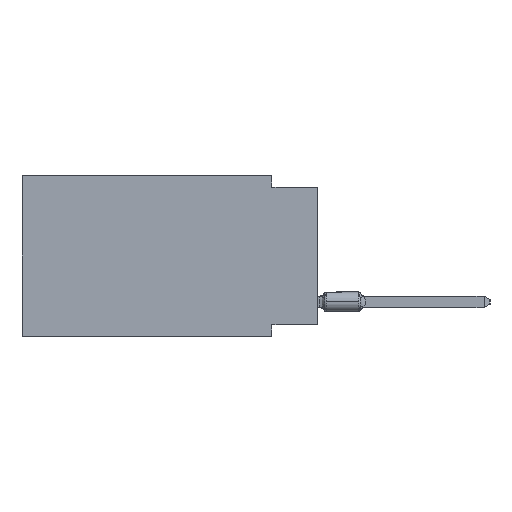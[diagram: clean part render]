
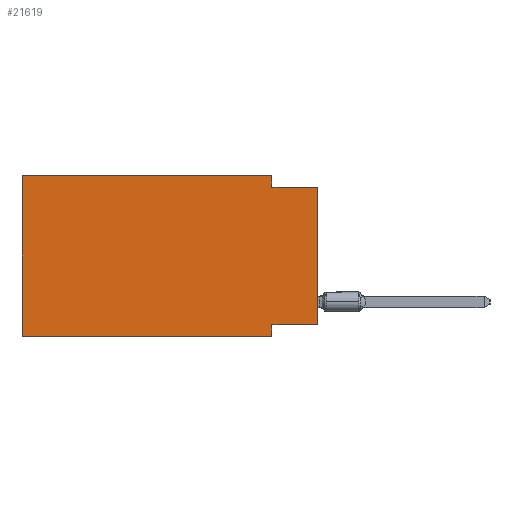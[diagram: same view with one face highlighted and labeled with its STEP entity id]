
A CAD part, left-side view. The second image highlights one B-rep face of the part: STEP entity #21619.
In plain terms, the highlighted planar face has unit normal (-1, 0, 0).
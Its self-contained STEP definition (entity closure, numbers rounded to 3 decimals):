
#1135 = VERTEX_POINT ( 'NONE', #19517 ) ;
#1807 = EDGE_CURVE ( 'NONE', #23763, #14638, #7992, .T. ) ;
#1973 = CARTESIAN_POINT ( 'NONE',  ( 0., 2.54, 0. ) ) ;
#2232 = FACE_OUTER_BOUND ( 'NONE', #28130, .T. ) ;
#3618 = DIRECTION ( 'NONE',  ( 0., 0., 1. ) ) ;
#3708 = DIRECTION ( 'NONE',  ( 0., 1., 0. ) ) ;
#3737 = VECTOR ( 'NONE', #17400, 1000. ) ;
#3788 = EDGE_CURVE ( 'NONE', #20009, #9669, #29826, .T. ) ;
#3922 = ORIENTED_EDGE ( 'NONE', *, *, #27219, .T. ) ;
#4349 = VERTEX_POINT ( 'NONE', #7233 ) ;
#4530 = ORIENTED_EDGE ( 'NONE', *, *, #3788, .T. ) ;
#4580 = VECTOR ( 'NONE', #27569, 1000. ) ;
#4931 = LINE ( 'NONE', #18668, #24850 ) ;
#5851 = VECTOR ( 'NONE', #3708, 1000. ) ;
#5910 = EDGE_CURVE ( 'NONE', #20009, #1135, #22518, .T. ) ;
#6583 = LINE ( 'NONE', #15995, #4580 ) ;
#7233 = CARTESIAN_POINT ( 'NONE',  ( 0., 2.54, -0.635 ) ) ;
#7331 = CARTESIAN_POINT ( 'NONE',  ( 0., 0., -8.255 ) ) ;
#7437 = ORIENTED_EDGE ( 'NONE', *, *, #1807, .F. ) ;
#7470 = ORIENTED_EDGE ( 'NONE', *, *, #5910, .F. ) ;
#7666 = CARTESIAN_POINT ( 'NONE',  ( 0., 16.383, 0. ) ) ;
#7992 = LINE ( 'NONE', #21720, #3737 ) ;
#8049 = ORIENTED_EDGE ( 'NONE', *, *, #16594, .F. ) ;
#8722 = LINE ( 'NONE', #25518, #11595 ) ;
#9015 = EDGE_CURVE ( 'NONE', #22147, #23763, #10734, .T. ) ;
#9669 = VERTEX_POINT ( 'NONE', #19572 ) ;
#10734 = LINE ( 'NONE', #7666, #14627 ) ;
#10968 = ORIENTED_EDGE ( 'NONE', *, *, #9015, .F. ) ;
#11595 = VECTOR ( 'NONE', #25662, 1000. ) ;
#11788 = DIRECTION ( 'NONE',  ( 1., 0., 0. ) ) ;
#12825 = EDGE_CURVE ( 'NONE', #4349, #9669, #13723, .T. ) ;
#13723 = LINE ( 'NONE', #23113, #22487 ) ;
#13924 = DIRECTION ( 'NONE',  ( 0., 0., -1. ) ) ;
#14014 = VERTEX_POINT ( 'NONE', #28874 ) ;
#14190 = DIRECTION ( 'NONE',  ( 0., -1., 0. ) ) ;
#14255 = ORIENTED_EDGE ( 'NONE', *, *, #12825, .F. ) ;
#14627 = VECTOR ( 'NONE', #17071, 1000. ) ;
#14638 = VERTEX_POINT ( 'NONE', #1973 ) ;
#15995 = CARTESIAN_POINT ( 'NONE',  ( 0., 2.54, -8.89 ) ) ;
#16594 = EDGE_CURVE ( 'NONE', #14638, #4349, #4931, .T. ) ;
#17071 = DIRECTION ( 'NONE',  ( 0., 0., 1. ) ) ;
#17400 = DIRECTION ( 'NONE',  ( 0., -1., 0. ) ) ;
#18668 = CARTESIAN_POINT ( 'NONE',  ( 0., 2.54, 0. ) ) ;
#19454 = CARTESIAN_POINT ( 'NONE',  ( 0., 16.383, -8.89 ) ) ;
#19517 = CARTESIAN_POINT ( 'NONE',  ( 0., 2.54, -8.255 ) ) ;
#19572 = CARTESIAN_POINT ( 'NONE',  ( 0., 0., -0.635 ) ) ;
#20009 = VERTEX_POINT ( 'NONE', #7331 ) ;
#20565 = PLANE ( 'NONE',  #21254 ) ;
#21254 = AXIS2_PLACEMENT_3D ( 'NONE', #23502, #11788, #13924 ) ;
#21619 = ADVANCED_FACE ( 'NONE', ( #2232 ), #20565, .F. ) ;
#21720 = CARTESIAN_POINT ( 'NONE',  ( 0., 16.383, 0. ) ) ;
#22147 = VERTEX_POINT ( 'NONE', #19454 ) ;
#22487 = VECTOR ( 'NONE', #14190, 1000. ) ;
#22518 = LINE ( 'NONE', #24671, #5851 ) ;
#22722 = CARTESIAN_POINT ( 'NONE',  ( 0., 0., 0. ) ) ;
#23113 = CARTESIAN_POINT ( 'NONE',  ( 0., 0., -0.635 ) ) ;
#23502 = CARTESIAN_POINT ( 'NONE',  ( 0., 16.383, 0. ) ) ;
#23763 = VERTEX_POINT ( 'NONE', #27431 ) ;
#24368 = VECTOR ( 'NONE', #3618, 1000. ) ;
#24671 = CARTESIAN_POINT ( 'NONE',  ( 0., 0., -8.255 ) ) ;
#24819 = ORIENTED_EDGE ( 'NONE', *, *, #25595, .F. ) ;
#24850 = VECTOR ( 'NONE', #28077, 1000. ) ;
#25518 = CARTESIAN_POINT ( 'NONE',  ( 0., 16.383, -8.89 ) ) ;
#25595 = EDGE_CURVE ( 'NONE', #1135, #14014, #6583, .T. ) ;
#25662 = DIRECTION ( 'NONE',  ( 0., -1., 0. ) ) ;
#27219 = EDGE_CURVE ( 'NONE', #22147, #14014, #8722, .T. ) ;
#27431 = CARTESIAN_POINT ( 'NONE',  ( 0., 16.383, 0. ) ) ;
#27569 = DIRECTION ( 'NONE',  ( 0., 0., -1. ) ) ;
#28077 = DIRECTION ( 'NONE',  ( 0., 0., -1. ) ) ;
#28130 = EDGE_LOOP ( 'NONE', ( #4530, #14255, #8049, #7437, #10968, #3922, #24819, #7470 ) ) ;
#28874 = CARTESIAN_POINT ( 'NONE',  ( 0., 2.54, -8.89 ) ) ;
#29826 = LINE ( 'NONE', #22722, #24368 ) ;
